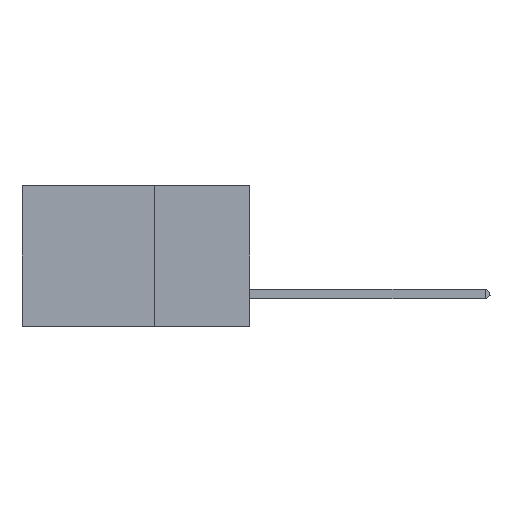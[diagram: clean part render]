
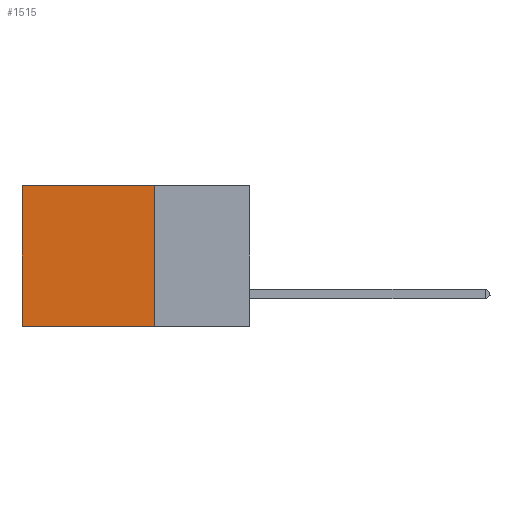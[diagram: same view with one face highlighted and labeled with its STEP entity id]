
A CAD part, left-side view. The second image highlights one B-rep face of the part: STEP entity #1515.
In plain terms, the highlighted planar face has unit normal (-1, 0, 0).
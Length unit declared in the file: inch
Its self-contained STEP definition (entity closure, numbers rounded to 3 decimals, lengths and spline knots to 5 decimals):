
#215 = EDGE_CURVE ( 'NONE', #4347, #5610, #21078, .T. ) ;
#915 = CARTESIAN_POINT ( 'NONE',  ( 0.2875, 0.6, 0. ) ) ;
#1515 = ADVANCED_FACE ( 'NONE', ( #20527 ), #24022, .F. ) ;
#1918 = VERTEX_POINT ( 'NONE', #915 ) ;
#2722 = VECTOR ( 'NONE', #18018, 39.37008 ) ;
#4347 = VERTEX_POINT ( 'NONE', #35518 ) ;
#4692 = LINE ( 'NONE', #35753, #27811 ) ;
#5610 = VERTEX_POINT ( 'NONE', #20122 ) ;
#5953 = VERTEX_POINT ( 'NONE', #38839 ) ;
#8641 = EDGE_CURVE ( 'NONE', #5953, #1918, #4692, .T. ) ;
#11458 = DIRECTION ( 'NONE',  ( 0., 0., -1. ) ) ;
#11514 = LINE ( 'NONE', #23818, #25250 ) ;
#11942 = CARTESIAN_POINT ( 'NONE',  ( 0.2875, 0.25, -0.37 ) ) ;
#13766 = DIRECTION ( 'NONE',  ( 0., 0., -1. ) ) ;
#13891 = CARTESIAN_POINT ( 'NONE',  ( 0.2875, 0.25, 0. ) ) ;
#15012 = VECTOR ( 'NONE', #13766, 39.37008 ) ;
#18018 = DIRECTION ( 'NONE',  ( 0., 1., 0. ) ) ;
#18330 = LINE ( 'NONE', #13891, #15012 ) ;
#18634 = ORIENTED_EDGE ( 'NONE', *, *, #21098, .F. ) ;
#19937 = DIRECTION ( 'NONE',  ( 1., 0., 0. ) ) ;
#20122 = CARTESIAN_POINT ( 'NONE',  ( 0.2875, 0.6, -0.37 ) ) ;
#20527 = FACE_OUTER_BOUND ( 'NONE', #26209, .T. ) ;
#21078 = LINE ( 'NONE', #11942, #2722 ) ;
#21098 = EDGE_CURVE ( 'NONE', #5953, #4347, #18330, .T. ) ;
#21747 = ORIENTED_EDGE ( 'NONE', *, *, #8641, .T. ) ;
#23818 = CARTESIAN_POINT ( 'NONE',  ( 0.2875, 0.6, 0. ) ) ;
#24022 = PLANE ( 'NONE',  #34100 ) ;
#25031 = ORIENTED_EDGE ( 'NONE', *, *, #28712, .T. ) ;
#25250 = VECTOR ( 'NONE', #32734, 39.37008 ) ;
#26105 = ORIENTED_EDGE ( 'NONE', *, *, #215, .F. ) ;
#26209 = EDGE_LOOP ( 'NONE', ( #25031, #26105, #18634, #21747 ) ) ;
#27811 = VECTOR ( 'NONE', #33249, 39.37008 ) ;
#28712 = EDGE_CURVE ( 'NONE', #1918, #5610, #11514, .T. ) ;
#32734 = DIRECTION ( 'NONE',  ( 0., 0., -1. ) ) ;
#33249 = DIRECTION ( 'NONE',  ( 0., 1., 0. ) ) ;
#34100 = AXIS2_PLACEMENT_3D ( 'NONE', #37147, #19937, #11458 ) ;
#35518 = CARTESIAN_POINT ( 'NONE',  ( 0.2875, 0.25, -0.37 ) ) ;
#35753 = CARTESIAN_POINT ( 'NONE',  ( 0.2875, 0.25, 0. ) ) ;
#37147 = CARTESIAN_POINT ( 'NONE',  ( 0.2875, 0.25, 0. ) ) ;
#38839 = CARTESIAN_POINT ( 'NONE',  ( 0.2875, 0.25, 0. ) ) ;
